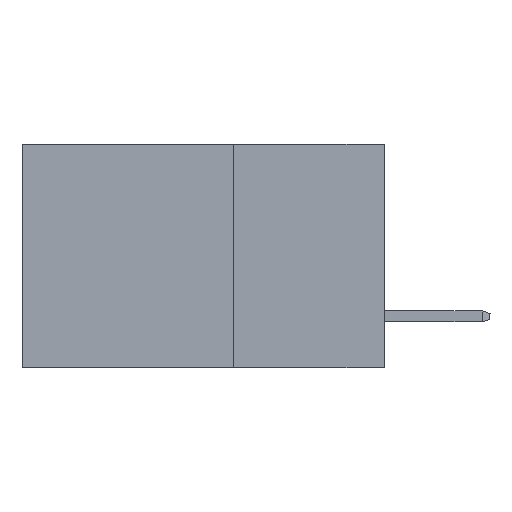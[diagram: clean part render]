
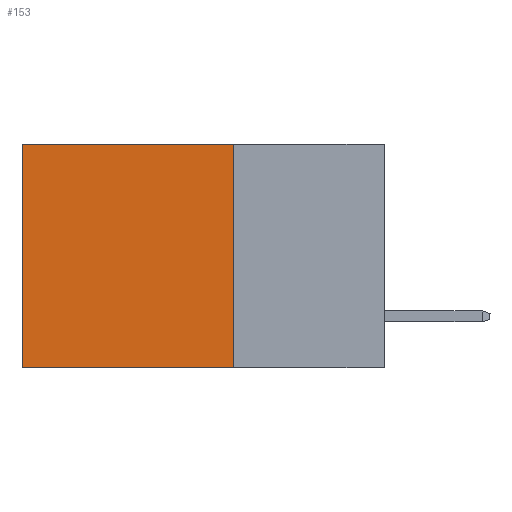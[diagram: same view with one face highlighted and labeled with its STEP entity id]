
A CAD part, left-side view. The second image highlights one B-rep face of the part: STEP entity #153.
In plain terms, the highlighted planar face has unit normal (-1, 0, 0).
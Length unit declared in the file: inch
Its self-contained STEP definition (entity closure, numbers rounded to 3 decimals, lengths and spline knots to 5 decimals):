
#77 = ORIENTED_EDGE ( 'NONE', *, *, #816, .T. ) ;
#153 = ADVANCED_FACE ( 'NONE', ( #6212 ), #8103, .F. ) ;
#434 = LINE ( 'NONE', #6666, #7060 ) ;
#816 = EDGE_CURVE ( 'NONE', #3032, #5024, #1029, .T. ) ;
#1029 = LINE ( 'NONE', #2440, #1284 ) ;
#1083 = CARTESIAN_POINT ( 'NONE',  ( 0.2615, 0.25, -0.37 ) ) ;
#1284 = VECTOR ( 'NONE', #3772, 39.37008 ) ;
#1779 = CARTESIAN_POINT ( 'NONE',  ( 0.2615, 0.25, 0. ) ) ;
#2354 = EDGE_CURVE ( 'NONE', #5024, #8668, #6048, .T. ) ;
#2440 = CARTESIAN_POINT ( 'NONE',  ( 0.2615, 0.25, 0. ) ) ;
#2473 = CARTESIAN_POINT ( 'NONE',  ( 0.2615, 0.25, -0.37 ) ) ;
#2610 = CARTESIAN_POINT ( 'NONE',  ( 0.2615, 0.25, -0.37 ) ) ;
#3032 = VERTEX_POINT ( 'NONE', #1779 ) ;
#3240 = ORIENTED_EDGE ( 'NONE', *, *, #4153, .F. ) ;
#3680 = ORIENTED_EDGE ( 'NONE', *, *, #2354, .T. ) ;
#3772 = DIRECTION ( 'NONE',  ( 0., 1., 0. ) ) ;
#4153 = EDGE_CURVE ( 'NONE', #8142, #8668, #8277, .T. ) ;
#4565 = VECTOR ( 'NONE', #7483, 39.37008 ) ;
#5022 = AXIS2_PLACEMENT_3D ( 'NONE', #2473, #5278, #5801 ) ;
#5024 = VERTEX_POINT ( 'NONE', #6783 ) ;
#5278 = DIRECTION ( 'NONE',  ( 1., 0., 0. ) ) ;
#5374 = DIRECTION ( 'NONE',  ( 0., 1., 0. ) ) ;
#5382 = CARTESIAN_POINT ( 'NONE',  ( 0.2615, 0.6, -0.37 ) ) ;
#5666 = EDGE_LOOP ( 'NONE', ( #3680, #3240, #8879, #77 ) ) ;
#5680 = EDGE_CURVE ( 'NONE', #3032, #8142, #434, .T. ) ;
#5801 = DIRECTION ( 'NONE',  ( 0., 0., -1. ) ) ;
#6048 = LINE ( 'NONE', #5382, #4565 ) ;
#6212 = FACE_OUTER_BOUND ( 'NONE', #5666, .T. ) ;
#6368 = VECTOR ( 'NONE', #5374, 39.37008 ) ;
#6666 = CARTESIAN_POINT ( 'NONE',  ( 0.2615, 0.25, -0.37 ) ) ;
#6708 = DIRECTION ( 'NONE',  ( 0., 0., -1. ) ) ;
#6783 = CARTESIAN_POINT ( 'NONE',  ( 0.2615, 0.6, 0. ) ) ;
#7060 = VECTOR ( 'NONE', #6708, 39.37008 ) ;
#7483 = DIRECTION ( 'NONE',  ( 0., 0., -1. ) ) ;
#7525 = CARTESIAN_POINT ( 'NONE',  ( 0.2615, 0.6, -0.37 ) ) ;
#8103 = PLANE ( 'NONE',  #5022 ) ;
#8142 = VERTEX_POINT ( 'NONE', #1083 ) ;
#8277 = LINE ( 'NONE', #2610, #6368 ) ;
#8668 = VERTEX_POINT ( 'NONE', #7525 ) ;
#8879 = ORIENTED_EDGE ( 'NONE', *, *, #5680, .F. ) ;
